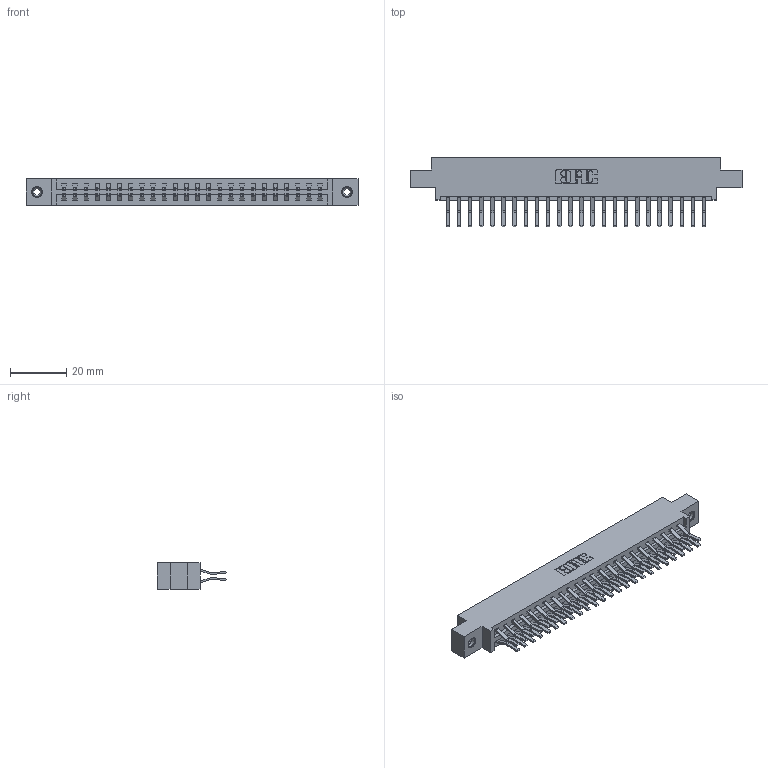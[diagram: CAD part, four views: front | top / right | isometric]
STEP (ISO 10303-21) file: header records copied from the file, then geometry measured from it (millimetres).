
FILE_DESCRIPTION (( 'STEP AP203' ), '1' );
FILE_NAME ('337-048-560-808.STEP', '2019-10-11T17:15:30', ( '' ), ( '' ), 'SwSTEP 2.0', 'SolidWorks 2016', '' );
FILE_SCHEMA (( 'CONFIG_CONTROL_DESIGN' ));
Length unit declared in the file: inch
Products named in the file (4): 337 Part_0.170 Offset - 0.156 Dia-TI; 345-250-001_345-250-003-102; 345-292-001_560 Tail; 337-048-560-808
Assembly tree (51 placements, depth 2):
  337-048-560-808
    337 Part_0.170 Offset - 0.156 Dia-TI
    345-292-001_560 Tail  x48
    345-250-001_345-250-003-102  x2
Bounding box: 118.11 x 24.78 x 9.4 mm (x, y, z)
Volume: 12398.4 mm3; surface area: 14883.9 mm2
Topology: 51 solids, 51 shells, 2866 faces, 8475 edges, 5578 vertices
Faces by surface type: plane 1930, cylinder 920, cone 12, torus 4
Entity records: 22342 total; most frequent: CARTESIAN_POINT 3761, ORIENTED_EDGE 3690, DIRECTION 3267, EDGE_CURVE 1845, VECTOR 1693, LINE 1693, VERTEX_POINT 1224, AXIS2_PLACEMENT_3D 787
